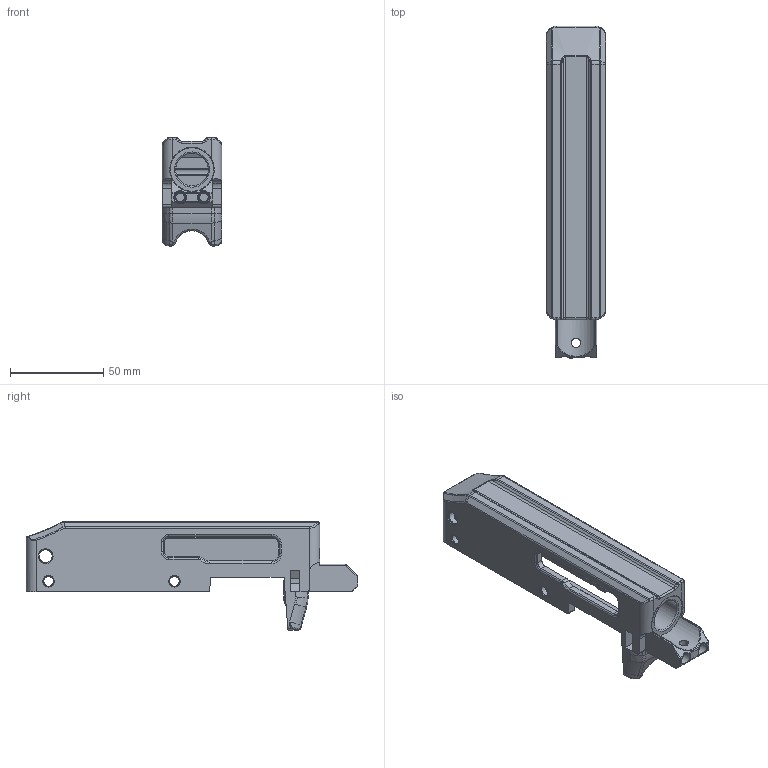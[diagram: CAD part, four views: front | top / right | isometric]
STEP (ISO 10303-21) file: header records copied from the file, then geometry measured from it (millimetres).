
FILE_DESCRIPTION(/* description */ (''),/* implementation_level */ '2;1');
FILE_NAME(/* name */ 'L-X22 Model I-R.step',/* time_stamp */ '2021-08-08T17:00:55-04:00',/* author */ (''),/* organization */ (''),/* preprocessor_version */ 'ST-DEVELOPER v18.1',/* originating_system */ 'Autodesk Translation Framework v10.9.0.1377',/* authorisation */ '');
FILE_SCHEMA (('AUTOMOTIVE_DESIGN { 1 0 10303 214 3 1 1 }'));
Length unit declared in the file: millimetre
Products named in the file (1): LX22 Model I-R Receiver
Bounding box: 31.95 x 177.8 x 58.08 mm (x, y, z)
Volume: 79086.1 mm3; surface area: 35874.8 mm2
Topology: 1 solids, 1 shells, 413 faces, 1069 edges, 646 vertices
Faces by surface type: cylinder 124, bspline 109, plane 104, torus 48, cone 22, sphere 6
Full cylindrical faces by diameter (mm): 1.6 x1, 4.648 x4, 5 x1, 5.175 x4, 6.426 x2, 6.95 x1, 15.6 x1, 17.45 x1, 23.393 x1
Entity records: 15469 total; most frequent: CARTESIAN_POINT 5801, ORIENTED_EDGE 2114, DIRECTION 1907, EDGE_CURVE 1057, AXIS2_PLACEMENT_3D 749, VERTEX_POINT 646, EDGE_LOOP 439, FACE_OUTER_BOUND 413
